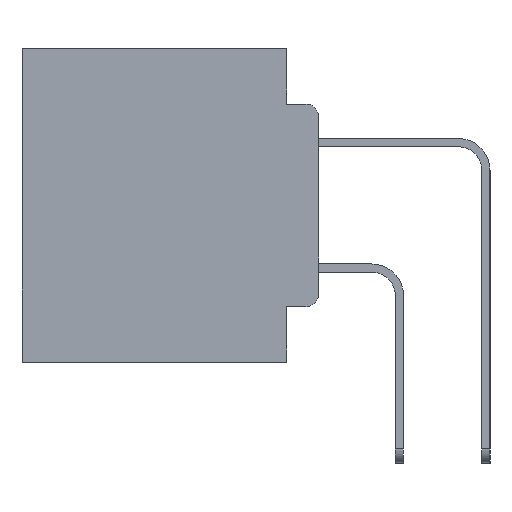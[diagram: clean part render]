
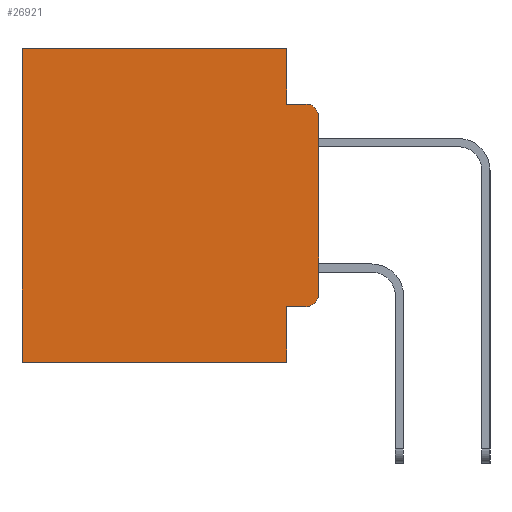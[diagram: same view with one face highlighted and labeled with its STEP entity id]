
A CAD part, left-side view. The second image highlights one B-rep face of the part: STEP entity #26921.
In plain terms, the highlighted planar face has unit normal (-1, 0, 0).
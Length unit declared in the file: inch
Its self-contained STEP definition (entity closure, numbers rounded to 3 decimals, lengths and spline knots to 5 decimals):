
#82 = ORIENTED_EDGE ( 'NONE', *, *, #15712, .F. ) ;
#97 = CARTESIAN_POINT ( 'NONE',  ( 0.298, 0.473, -0.5 ) ) ;
#738 = CARTESIAN_POINT ( 'NONE',  ( 0.298, 0.02, -0.3915 ) ) ;
#1238 = CARTESIAN_POINT ( 'NONE',  ( 0.298, 0.02, -0.1085 ) ) ;
#1730 = AXIS2_PLACEMENT_3D ( 'NONE', #1238, #18443, #17933 ) ;
#2041 = DIRECTION ( 'NONE',  ( 0., 0., -1. ) ) ;
#2125 = CARTESIAN_POINT ( 'NONE',  ( 0.298, 0., -0.3915 ) ) ;
#2292 = CARTESIAN_POINT ( 'NONE',  ( 0.298, 0., -0.5 ) ) ;
#2428 = EDGE_LOOP ( 'NONE', ( #82, #16945, #24049, #15160, #24720, #12060, #21677, #24436, #23768, #8108 ) ) ;
#3013 = DIRECTION ( 'NONE',  ( 0., 0., -1. ) ) ;
#3392 = DIRECTION ( 'NONE',  ( 0., 1., 0. ) ) ;
#3413 = EDGE_CURVE ( 'NONE', #28427, #7723, #21996, .T. ) ;
#3721 = CARTESIAN_POINT ( 'NONE',  ( 0.298, 0., -0.1085 ) ) ;
#4537 = CARTESIAN_POINT ( 'NONE',  ( 0.298, 0.051, 0. ) ) ;
#4609 = DIRECTION ( 'NONE',  ( 0., 1., 0. ) ) ;
#4982 = EDGE_CURVE ( 'NONE', #11141, #7304, #12615, .T. ) ;
#6186 = VECTOR ( 'NONE', #15438, 39.37008 ) ;
#6842 = CARTESIAN_POINT ( 'NONE',  ( 0.298, 0., 0. ) ) ;
#7304 = VERTEX_POINT ( 'NONE', #97 ) ;
#7605 = EDGE_CURVE ( 'NONE', #28055, #20403, #19748, .T. ) ;
#7723 = VERTEX_POINT ( 'NONE', #28290 ) ;
#7864 = VERTEX_POINT ( 'NONE', #22379 ) ;
#8038 = CARTESIAN_POINT ( 'NONE',  ( 0.298, 0., 0. ) ) ;
#8108 = ORIENTED_EDGE ( 'NONE', *, *, #19751, .T. ) ;
#8278 = DIRECTION ( 'NONE',  ( 0., 0., -1. ) ) ;
#8421 = VECTOR ( 'NONE', #21511, 39.37008 ) ;
#8514 = AXIS2_PLACEMENT_3D ( 'NONE', #6842, #22492, #9209 ) ;
#9209 = DIRECTION ( 'NONE',  ( 0., 0., -1. ) ) ;
#9227 = VECTOR ( 'NONE', #20292, 39.37008 ) ;
#9258 = VECTOR ( 'NONE', #8278, 39.37008 ) ;
#9848 = CARTESIAN_POINT ( 'NONE',  ( 0.298, 0.473, 0. ) ) ;
#10967 = VERTEX_POINT ( 'NONE', #27376 ) ;
#11141 = VERTEX_POINT ( 'NONE', #25784 ) ;
#11419 = EDGE_CURVE ( 'NONE', #20403, #7304, #26284, .T. ) ;
#11636 = LINE ( 'NONE', #28425, #6186 ) ;
#12035 = AXIS2_PLACEMENT_3D ( 'NONE', #738, #16708, #3013 ) ;
#12060 = ORIENTED_EDGE ( 'NONE', *, *, #11419, .T. ) ;
#12108 = CARTESIAN_POINT ( 'NONE',  ( 0.298, 0.051, -0.4115 ) ) ;
#12245 = VECTOR ( 'NONE', #23097, 39.37008 ) ;
#12615 = LINE ( 'NONE', #2292, #23623 ) ;
#14726 = VECTOR ( 'NONE', #2041, 39.37008 ) ;
#14765 = EDGE_CURVE ( 'NONE', #28889, #11141, #21051, .T. ) ;
#15160 = ORIENTED_EDGE ( 'NONE', *, *, #25000, .F. ) ;
#15438 = DIRECTION ( 'NONE',  ( 0., -1., 0. ) ) ;
#15712 = EDGE_CURVE ( 'NONE', #28427, #25762, #19613, .T. ) ;
#16234 = EDGE_CURVE ( 'NONE', #10967, #7723, #11636, .T. ) ;
#16708 = DIRECTION ( 'NONE',  ( -1., 0., 0. ) ) ;
#16945 = ORIENTED_EDGE ( 'NONE', *, *, #3413, .T. ) ;
#17933 = DIRECTION ( 'NONE',  ( 0., 0., -1. ) ) ;
#18084 = PLANE ( 'NONE',  #8514 ) ;
#18096 = CARTESIAN_POINT ( 'NONE',  ( 0.298, 0.051, 0. ) ) ;
#18443 = DIRECTION ( 'NONE',  ( -1., 0., 0. ) ) ;
#18809 = LINE ( 'NONE', #20894, #12245 ) ;
#19074 = VECTOR ( 'NONE', #3392, 39.37008 ) ;
#19613 = LINE ( 'NONE', #8038, #8421 ) ;
#19748 = LINE ( 'NONE', #25701, #19074 ) ;
#19751 = EDGE_CURVE ( 'NONE', #7864, #25762, #24198, .T. ) ;
#20292 = DIRECTION ( 'NONE',  ( 0., 0., -1. ) ) ;
#20403 = VERTEX_POINT ( 'NONE', #9848 ) ;
#20894 = CARTESIAN_POINT ( 'NONE',  ( 0.298, 0.051, -0.4115 ) ) ;
#21051 = LINE ( 'NONE', #18096, #9227 ) ;
#21087 = LINE ( 'NONE', #23839, #9258 ) ;
#21511 = DIRECTION ( 'NONE',  ( 0., 0., -1. ) ) ;
#21677 = ORIENTED_EDGE ( 'NONE', *, *, #4982, .F. ) ;
#21996 = CIRCLE ( 'NONE', #1730, 0.02 ) ;
#22379 = CARTESIAN_POINT ( 'NONE',  ( 0.298, 0.02, -0.4115 ) ) ;
#22492 = DIRECTION ( 'NONE',  ( 1., 0., 0. ) ) ;
#23097 = DIRECTION ( 'NONE',  ( 0., -1., 0. ) ) ;
#23623 = VECTOR ( 'NONE', #4609, 39.37008 ) ;
#23768 = ORIENTED_EDGE ( 'NONE', *, *, #26420, .T. ) ;
#23839 = CARTESIAN_POINT ( 'NONE',  ( 0.298, 0.051, 0. ) ) ;
#24049 = ORIENTED_EDGE ( 'NONE', *, *, #16234, .F. ) ;
#24198 = CIRCLE ( 'NONE', #12035, 0.02 ) ;
#24436 = ORIENTED_EDGE ( 'NONE', *, *, #14765, .F. ) ;
#24720 = ORIENTED_EDGE ( 'NONE', *, *, #7605, .T. ) ;
#25000 = EDGE_CURVE ( 'NONE', #28055, #10967, #21087, .T. ) ;
#25701 = CARTESIAN_POINT ( 'NONE',  ( 0.298, 0., 0. ) ) ;
#25762 = VERTEX_POINT ( 'NONE', #2125 ) ;
#25784 = CARTESIAN_POINT ( 'NONE',  ( 0.298, 0.051, -0.5 ) ) ;
#26284 = LINE ( 'NONE', #26595, #14726 ) ;
#26420 = EDGE_CURVE ( 'NONE', #28889, #7864, #18809, .T. ) ;
#26595 = CARTESIAN_POINT ( 'NONE',  ( 0.298, 0.473, 0. ) ) ;
#26921 = ADVANCED_FACE ( 'NONE', ( #28905 ), #18084, .F. ) ;
#27376 = CARTESIAN_POINT ( 'NONE',  ( 0.298, 0.051, -0.0885 ) ) ;
#28055 = VERTEX_POINT ( 'NONE', #4537 ) ;
#28290 = CARTESIAN_POINT ( 'NONE',  ( 0.298, 0.02, -0.0885 ) ) ;
#28425 = CARTESIAN_POINT ( 'NONE',  ( 0.298, 0.051, -0.0885 ) ) ;
#28427 = VERTEX_POINT ( 'NONE', #3721 ) ;
#28889 = VERTEX_POINT ( 'NONE', #12108 ) ;
#28905 = FACE_OUTER_BOUND ( 'NONE', #2428, .T. ) ;
